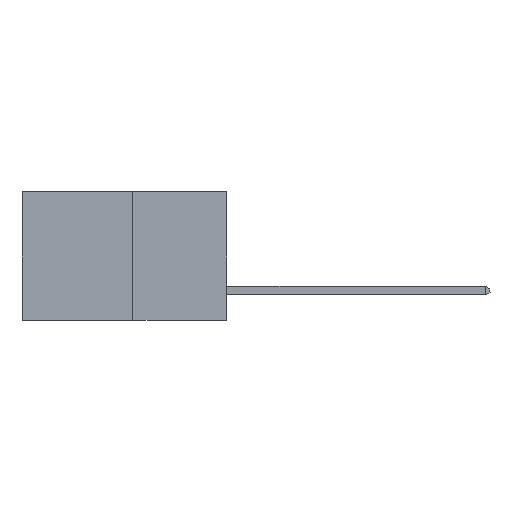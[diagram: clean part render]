
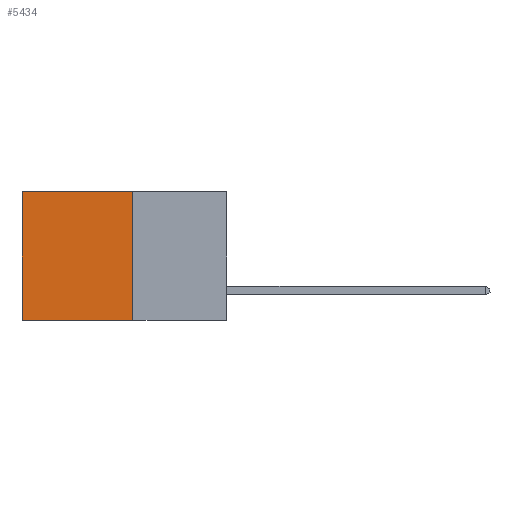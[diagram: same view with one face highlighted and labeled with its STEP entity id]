
A CAD part, left-side view. The second image highlights one B-rep face of the part: STEP entity #5434.
In plain terms, the highlighted planar face has unit normal (-1, 0, 0).
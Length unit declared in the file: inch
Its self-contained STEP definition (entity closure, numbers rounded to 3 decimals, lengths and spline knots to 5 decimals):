
#274 = EDGE_LOOP ( 'NONE', ( #1288, #3220, #2446, #8303 ) ) ;
#439 = LINE ( 'NONE', #7754, #6093 ) ;
#1288 = ORIENTED_EDGE ( 'NONE', *, *, #5251, .T. ) ;
#2446 = ORIENTED_EDGE ( 'NONE', *, *, #3317, .F. ) ;
#2463 = LINE ( 'NONE', #7431, #4709 ) ;
#3041 = VERTEX_POINT ( 'NONE', #6962 ) ;
#3200 = VECTOR ( 'NONE', #7214, 39.37008 ) ;
#3220 = ORIENTED_EDGE ( 'NONE', *, *, #4262, .F. ) ;
#3317 = EDGE_CURVE ( 'NONE', #5658, #5952, #4039, .T. ) ;
#3433 = LINE ( 'NONE', #7233, #3200 ) ;
#3793 = FACE_OUTER_BOUND ( 'NONE', #274, .T. ) ;
#3947 = CARTESIAN_POINT ( 'NONE',  ( 0.277, 0.27, -0.37 ) ) ;
#4039 = LINE ( 'NONE', #8634, #5938 ) ;
#4262 = EDGE_CURVE ( 'NONE', #5952, #3041, #2463, .T. ) ;
#4513 = CARTESIAN_POINT ( 'NONE',  ( 0.277, 0.59, 0. ) ) ;
#4709 = VECTOR ( 'NONE', #7455, 39.37008 ) ;
#5251 = EDGE_CURVE ( 'NONE', #5843, #3041, #3433, .T. ) ;
#5302 = CARTESIAN_POINT ( 'NONE',  ( 0.277, 0.27, 0. ) ) ;
#5434 = ADVANCED_FACE ( 'NONE', ( #3793 ), #6530, .F. ) ;
#5658 = VERTEX_POINT ( 'NONE', #5302 ) ;
#5729 = DIRECTION ( 'NONE',  ( 0., 1., 0. ) ) ;
#5843 = VERTEX_POINT ( 'NONE', #4513 ) ;
#5938 = VECTOR ( 'NONE', #8642, 39.37008 ) ;
#5952 = VERTEX_POINT ( 'NONE', #3947 ) ;
#6093 = VECTOR ( 'NONE', #5729, 39.37008 ) ;
#6190 = AXIS2_PLACEMENT_3D ( 'NONE', #6494, #6468, #6459 ) ;
#6459 = DIRECTION ( 'NONE',  ( 0., 0., -1. ) ) ;
#6468 = DIRECTION ( 'NONE',  ( 1., 0., 0. ) ) ;
#6494 = CARTESIAN_POINT ( 'NONE',  ( 0.277, 0.27, -0.37 ) ) ;
#6530 = PLANE ( 'NONE',  #6190 ) ;
#6856 = EDGE_CURVE ( 'NONE', #5658, #5843, #439, .T. ) ;
#6962 = CARTESIAN_POINT ( 'NONE',  ( 0.277, 0.59, -0.37 ) ) ;
#7214 = DIRECTION ( 'NONE',  ( 0., 0., -1. ) ) ;
#7233 = CARTESIAN_POINT ( 'NONE',  ( 0.277, 0.59, -0.37 ) ) ;
#7431 = CARTESIAN_POINT ( 'NONE',  ( 0.277, 0.27, -0.37 ) ) ;
#7455 = DIRECTION ( 'NONE',  ( 0., 1., 0. ) ) ;
#7754 = CARTESIAN_POINT ( 'NONE',  ( 0.277, 0.27, 0. ) ) ;
#8303 = ORIENTED_EDGE ( 'NONE', *, *, #6856, .T. ) ;
#8634 = CARTESIAN_POINT ( 'NONE',  ( 0.277, 0.27, -0.37 ) ) ;
#8642 = DIRECTION ( 'NONE',  ( 0., 0., -1. ) ) ;
